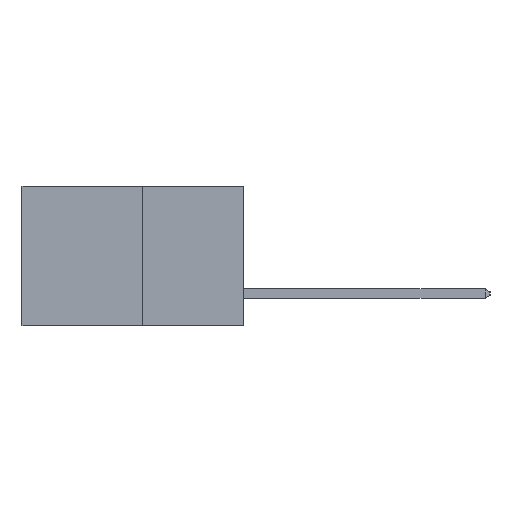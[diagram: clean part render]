
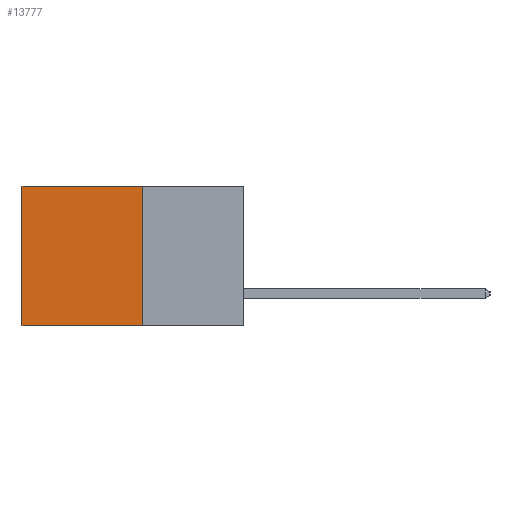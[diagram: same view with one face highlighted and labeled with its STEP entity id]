
A CAD part, left-side view. The second image highlights one B-rep face of the part: STEP entity #13777.
In plain terms, the highlighted planar face has unit normal (-1, 0, 0).
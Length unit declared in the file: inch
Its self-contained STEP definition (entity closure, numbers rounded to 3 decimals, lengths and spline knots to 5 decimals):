
#953 = DIRECTION ( 'NONE',  ( 0., 1., 0. ) ) ;
#976 = CARTESIAN_POINT ( 'NONE',  ( 0.277, 0.27, -0.37 ) ) ;
#1155 = CARTESIAN_POINT ( 'NONE',  ( 0.277, 0.27, 0. ) ) ;
#1547 = VERTEX_POINT ( 'NONE', #7967 ) ;
#1918 = EDGE_CURVE ( 'NONE', #9582, #5486, #12545, .T. ) ;
#2097 = EDGE_CURVE ( 'NONE', #5486, #8231, #10036, .T. ) ;
#2305 = CARTESIAN_POINT ( 'NONE',  ( 0.277, 0.27, -0.37 ) ) ;
#2876 = ORIENTED_EDGE ( 'NONE', *, *, #1918, .F. ) ;
#3044 = DIRECTION ( 'NONE',  ( 0., 0., -1. ) ) ;
#3110 = PLANE ( 'NONE',  #9739 ) ;
#3672 = EDGE_CURVE ( 'NONE', #9582, #1547, #6465, .T. ) ;
#3933 = VECTOR ( 'NONE', #953, 39.37008 ) ;
#4204 = FACE_OUTER_BOUND ( 'NONE', #4923, .T. ) ;
#4287 = CARTESIAN_POINT ( 'NONE',  ( 0.277, 0.27, -0.37 ) ) ;
#4923 = EDGE_LOOP ( 'NONE', ( #10623, #11723, #2876, #9012 ) ) ;
#5038 = DIRECTION ( 'NONE',  ( 0., 0., -1. ) ) ;
#5467 = DIRECTION ( 'NONE',  ( 1., 0., 0. ) ) ;
#5486 = VERTEX_POINT ( 'NONE', #14486 ) ;
#6465 = LINE ( 'NONE', #1155, #12146 ) ;
#6522 = VECTOR ( 'NONE', #5038, 39.37008 ) ;
#7967 = CARTESIAN_POINT ( 'NONE',  ( 0.277, 0.59, 0. ) ) ;
#8231 = VERTEX_POINT ( 'NONE', #8633 ) ;
#8633 = CARTESIAN_POINT ( 'NONE',  ( 0.277, 0.59, -0.37 ) ) ;
#9012 = ORIENTED_EDGE ( 'NONE', *, *, #3672, .T. ) ;
#9205 = LINE ( 'NONE', #11135, #12247 ) ;
#9582 = VERTEX_POINT ( 'NONE', #14620 ) ;
#9739 = AXIS2_PLACEMENT_3D ( 'NONE', #4287, #5467, #13419 ) ;
#10036 = LINE ( 'NONE', #2305, #3933 ) ;
#10623 = ORIENTED_EDGE ( 'NONE', *, *, #10657, .T. ) ;
#10657 = EDGE_CURVE ( 'NONE', #1547, #8231, #9205, .T. ) ;
#11135 = CARTESIAN_POINT ( 'NONE',  ( 0.277, 0.59, -0.37 ) ) ;
#11723 = ORIENTED_EDGE ( 'NONE', *, *, #2097, .F. ) ;
#12146 = VECTOR ( 'NONE', #12917, 39.37008 ) ;
#12247 = VECTOR ( 'NONE', #3044, 39.37008 ) ;
#12545 = LINE ( 'NONE', #976, #6522 ) ;
#12917 = DIRECTION ( 'NONE',  ( 0., 1., 0. ) ) ;
#13419 = DIRECTION ( 'NONE',  ( 0., 0., -1. ) ) ;
#13777 = ADVANCED_FACE ( 'NONE', ( #4204 ), #3110, .F. ) ;
#14486 = CARTESIAN_POINT ( 'NONE',  ( 0.277, 0.27, -0.37 ) ) ;
#14620 = CARTESIAN_POINT ( 'NONE',  ( 0.277, 0.27, 0. ) ) ;
